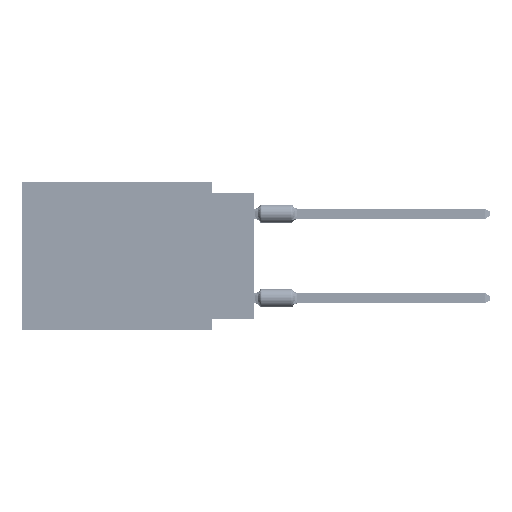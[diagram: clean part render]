
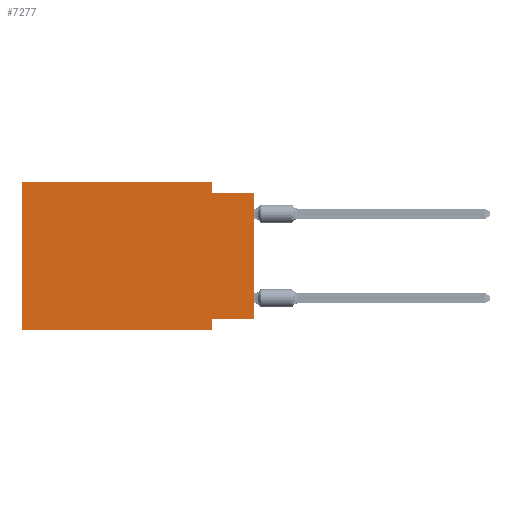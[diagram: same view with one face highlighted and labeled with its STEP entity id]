
A CAD part, left-side view. The second image highlights one B-rep face of the part: STEP entity #7277.
In plain terms, the highlighted planar face has unit normal (-1, 0, 0).
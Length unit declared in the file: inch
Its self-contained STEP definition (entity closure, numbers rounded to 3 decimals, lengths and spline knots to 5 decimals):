
#1143 = LINE ( 'NONE', #3225, #48248 ) ;
#1953 = ORIENTED_EDGE ( 'NONE', *, *, #27684, .F. ) ;
#2795 = DIRECTION ( 'NONE',  ( 0., 1., 0. ) ) ;
#3225 = CARTESIAN_POINT ( 'NONE',  ( 0., 0., 0. ) ) ;
#3494 = VECTOR ( 'NONE', #2795, 39.37008 ) ;
#6618 = CARTESIAN_POINT ( 'NONE',  ( 0., 0.1, 0. ) ) ;
#7277 = ADVANCED_FACE ( 'NONE', ( #42940 ), #8952, .F. ) ;
#7701 = DIRECTION ( 'NONE',  ( 0., -1., 0. ) ) ;
#8952 = PLANE ( 'NONE',  #27010 ) ;
#9057 = VERTEX_POINT ( 'NONE', #54857 ) ;
#9135 = VERTEX_POINT ( 'NONE', #30171 ) ;
#11160 = DIRECTION ( 'NONE',  ( 0., -1., 0. ) ) ;
#13085 = ORIENTED_EDGE ( 'NONE', *, *, #21363, .T. ) ;
#13339 = VECTOR ( 'NONE', #22085, 39.37008 ) ;
#13471 = EDGE_LOOP ( 'NONE', ( #79792, #1953, #24046, #42571, #80530, #13085, #60455, #53179 ) ) ;
#15706 = VECTOR ( 'NONE', #54415, 39.37008 ) ;
#20020 = CARTESIAN_POINT ( 'NONE',  ( 0., 0.1, -0.325 ) ) ;
#20930 = LINE ( 'NONE', #56000, #35981 ) ;
#21315 = CARTESIAN_POINT ( 'NONE',  ( 0., 0.55, 0. ) ) ;
#21363 = EDGE_CURVE ( 'NONE', #25471, #26462, #25556, .T. ) ;
#21536 = VECTOR ( 'NONE', #7701, 39.37008 ) ;
#22085 = DIRECTION ( 'NONE',  ( 0., -1., 0. ) ) ;
#24046 = ORIENTED_EDGE ( 'NONE', *, *, #36117, .F. ) ;
#25471 = VERTEX_POINT ( 'NONE', #57131 ) ;
#25556 = LINE ( 'NONE', #59007, #21536 ) ;
#26462 = VERTEX_POINT ( 'NONE', #46344 ) ;
#27010 = AXIS2_PLACEMENT_3D ( 'NONE', #34736, #79513, #41157 ) ;
#27684 = EDGE_CURVE ( 'NONE', #28491, #9135, #79491, .T. ) ;
#28491 = VERTEX_POINT ( 'NONE', #55037 ) ;
#30171 = CARTESIAN_POINT ( 'NONE',  ( 0., 0., -0.025 ) ) ;
#32041 = EDGE_CURVE ( 'NONE', #80715, #9135, #1143, .T. ) ;
#32762 = LINE ( 'NONE', #34823, #15706 ) ;
#34736 = CARTESIAN_POINT ( 'NONE',  ( 0., 0.55, 0. ) ) ;
#34823 = CARTESIAN_POINT ( 'NONE',  ( 0., 0.55, 0. ) ) ;
#34984 = CARTESIAN_POINT ( 'NONE',  ( 0., 0., -0.025 ) ) ;
#35060 = VERTEX_POINT ( 'NONE', #21315 ) ;
#35981 = VECTOR ( 'NONE', #11160, 39.37008 ) ;
#36117 = EDGE_CURVE ( 'NONE', #9057, #28491, #80086, .T. ) ;
#41157 = DIRECTION ( 'NONE',  ( 0., 0., -1. ) ) ;
#42571 = ORIENTED_EDGE ( 'NONE', *, *, #79408, .F. ) ;
#42940 = FACE_OUTER_BOUND ( 'NONE', #13471, .T. ) ;
#44978 = DIRECTION ( 'NONE',  ( 0., 0., -1. ) ) ;
#46019 = VECTOR ( 'NONE', #44978, 39.37008 ) ;
#46344 = CARTESIAN_POINT ( 'NONE',  ( 0., 0.1, -0.35 ) ) ;
#46600 = LINE ( 'NONE', #73040, #80660 ) ;
#48248 = VECTOR ( 'NONE', #67350, 39.37008 ) ;
#51324 = VERTEX_POINT ( 'NONE', #20020 ) ;
#53179 = ORIENTED_EDGE ( 'NONE', *, *, #81581, .F. ) ;
#54415 = DIRECTION ( 'NONE',  ( 0., 0., 1. ) ) ;
#54857 = CARTESIAN_POINT ( 'NONE',  ( 0., 0.1, 0. ) ) ;
#55037 = CARTESIAN_POINT ( 'NONE',  ( 0., 0.1, -0.025 ) ) ;
#56000 = CARTESIAN_POINT ( 'NONE',  ( 0., 0.55, 0. ) ) ;
#57131 = CARTESIAN_POINT ( 'NONE',  ( 0., 0.55, -0.35 ) ) ;
#59007 = CARTESIAN_POINT ( 'NONE',  ( 0., 0.55, -0.35 ) ) ;
#60455 = ORIENTED_EDGE ( 'NONE', *, *, #82809, .F. ) ;
#66650 = CARTESIAN_POINT ( 'NONE',  ( 0., 0., -0.325 ) ) ;
#67350 = DIRECTION ( 'NONE',  ( 0., 0., 1. ) ) ;
#69194 = CARTESIAN_POINT ( 'NONE',  ( 0., 0., -0.325 ) ) ;
#73040 = CARTESIAN_POINT ( 'NONE',  ( 0., 0.1, -0.35 ) ) ;
#79408 = EDGE_CURVE ( 'NONE', #35060, #9057, #20930, .T. ) ;
#79491 = LINE ( 'NONE', #34984, #13339 ) ;
#79513 = DIRECTION ( 'NONE',  ( 1., 0., 0. ) ) ;
#79792 = ORIENTED_EDGE ( 'NONE', *, *, #32041, .T. ) ;
#80038 = DIRECTION ( 'NONE',  ( 0., 0., -1. ) ) ;
#80086 = LINE ( 'NONE', #6618, #46019 ) ;
#80501 = EDGE_CURVE ( 'NONE', #25471, #35060, #32762, .T. ) ;
#80530 = ORIENTED_EDGE ( 'NONE', *, *, #80501, .F. ) ;
#80660 = VECTOR ( 'NONE', #80038, 39.37008 ) ;
#80715 = VERTEX_POINT ( 'NONE', #69194 ) ;
#81581 = EDGE_CURVE ( 'NONE', #80715, #51324, #82642, .T. ) ;
#82642 = LINE ( 'NONE', #66650, #3494 ) ;
#82809 = EDGE_CURVE ( 'NONE', #51324, #26462, #46600, .T. ) ;
